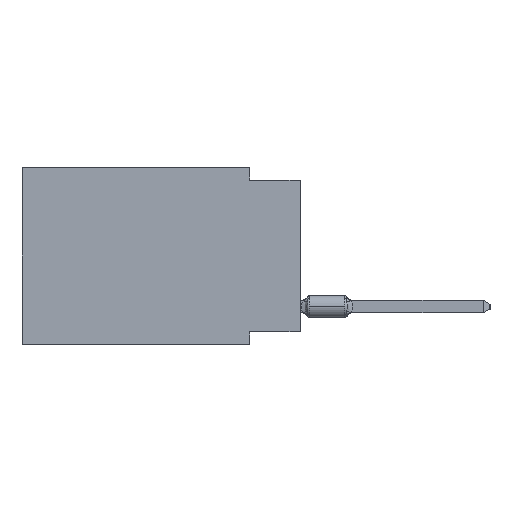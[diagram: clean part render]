
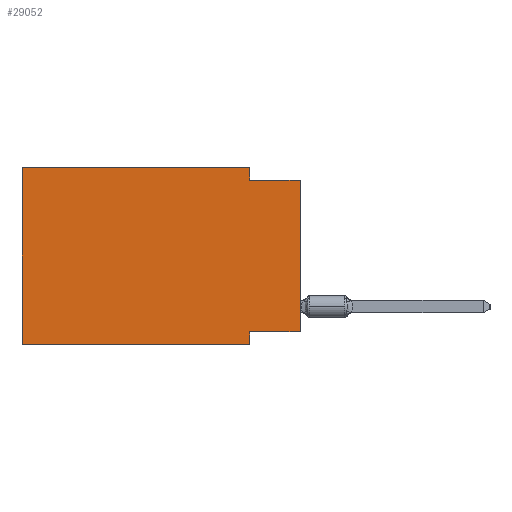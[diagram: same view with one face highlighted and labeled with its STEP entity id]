
A CAD part, left-side view. The second image highlights one B-rep face of the part: STEP entity #29052.
In plain terms, the highlighted planar face has unit normal (-1, 0, 0).
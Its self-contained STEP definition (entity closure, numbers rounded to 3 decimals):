
#316 = DIRECTION ( 'NONE',  ( 0., -1., 0. ) ) ;
#3468 = EDGE_CURVE ( 'NONE', #83949, #24442, #83530, .T. ) ;
#3730 = VERTEX_POINT ( 'NONE', #81602 ) ;
#4729 = EDGE_LOOP ( 'NONE', ( #78545, #19273, #7507, #60123, #86718, #85081, #77925, #61655 ) ) ;
#7156 = VERTEX_POINT ( 'NONE', #19546 ) ;
#7507 = ORIENTED_EDGE ( 'NONE', *, *, #25773, .F. ) ;
#7607 = EDGE_CURVE ( 'NONE', #8416, #3730, #48174, .T. ) ;
#8416 = VERTEX_POINT ( 'NONE', #82884 ) ;
#12441 = VECTOR ( 'NONE', #73471, 1000. ) ;
#12655 = EDGE_CURVE ( 'NONE', #71106, #7156, #22625, .T. ) ;
#12844 = CARTESIAN_POINT ( 'NONE',  ( 0., 2.54, -0.635 ) ) ;
#13614 = VECTOR ( 'NONE', #21148, 1000. ) ;
#15082 = CARTESIAN_POINT ( 'NONE',  ( 0., 0., -8.255 ) ) ;
#16675 = CARTESIAN_POINT ( 'NONE',  ( 0., 2.54, -8.89 ) ) ;
#18164 = LINE ( 'NONE', #24214, #45524 ) ;
#19273 = ORIENTED_EDGE ( 'NONE', *, *, #74665, .F. ) ;
#19546 = CARTESIAN_POINT ( 'NONE',  ( 0., 2.54, 0. ) ) ;
#21148 = DIRECTION ( 'NONE',  ( 0., 1., 0. ) ) ;
#21368 = VECTOR ( 'NONE', #70034, 1000. ) ;
#22625 = LINE ( 'NONE', #49651, #82276 ) ;
#22646 = FACE_OUTER_BOUND ( 'NONE', #4729, .T. ) ;
#23125 = PLANE ( 'NONE',  #54576 ) ;
#23143 = VECTOR ( 'NONE', #34197, 1000. ) ;
#23569 = CARTESIAN_POINT ( 'NONE',  ( 0., 13.97, 0. ) ) ;
#24214 = CARTESIAN_POINT ( 'NONE',  ( 0., 0., -0.635 ) ) ;
#24442 = VERTEX_POINT ( 'NONE', #63668 ) ;
#25773 = EDGE_CURVE ( 'NONE', #7156, #33038, #77188, .T. ) ;
#27216 = CARTESIAN_POINT ( 'NONE',  ( 0., 13.97, -8.89 ) ) ;
#29052 = ADVANCED_FACE ( 'NONE', ( #22646 ), #23125, .F. ) ;
#30479 = DIRECTION ( 'NONE',  ( 0., 0., 1. ) ) ;
#33038 = VERTEX_POINT ( 'NONE', #12844 ) ;
#34197 = DIRECTION ( 'NONE',  ( 0., -1., 0. ) ) ;
#37102 = DIRECTION ( 'NONE',  ( 0., 0., -1. ) ) ;
#41013 = CARTESIAN_POINT ( 'NONE',  ( 0., 0., -8.255 ) ) ;
#44602 = LINE ( 'NONE', #16675, #12441 ) ;
#45524 = VECTOR ( 'NONE', #53079, 1000. ) ;
#48174 = LINE ( 'NONE', #27216, #23143 ) ;
#49651 = CARTESIAN_POINT ( 'NONE',  ( 0., 13.97, 0. ) ) ;
#50788 = VERTEX_POINT ( 'NONE', #51064 ) ;
#51049 = DIRECTION ( 'NONE',  ( 1., 0., 0. ) ) ;
#51064 = CARTESIAN_POINT ( 'NONE',  ( 0., 2.54, -8.255 ) ) ;
#53079 = DIRECTION ( 'NONE',  ( 0., -1., 0. ) ) ;
#54576 = AXIS2_PLACEMENT_3D ( 'NONE', #23569, #51049, #79450 ) ;
#55616 = CARTESIAN_POINT ( 'NONE',  ( 0., 0., 0. ) ) ;
#58621 = VECTOR ( 'NONE', #37102, 1000. ) ;
#58983 = EDGE_CURVE ( 'NONE', #50788, #3730, #44602, .T. ) ;
#60123 = ORIENTED_EDGE ( 'NONE', *, *, #12655, .F. ) ;
#61453 = CARTESIAN_POINT ( 'NONE',  ( 0., 13.97, 0. ) ) ;
#61655 = ORIENTED_EDGE ( 'NONE', *, *, #79797, .F. ) ;
#63668 = CARTESIAN_POINT ( 'NONE',  ( 0., 0., -0.635 ) ) ;
#64074 = EDGE_CURVE ( 'NONE', #8416, #71106, #82098, .T. ) ;
#70034 = DIRECTION ( 'NONE',  ( 0., 0., 1. ) ) ;
#71106 = VERTEX_POINT ( 'NONE', #61453 ) ;
#73471 = DIRECTION ( 'NONE',  ( 0., 0., -1. ) ) ;
#74665 = EDGE_CURVE ( 'NONE', #33038, #24442, #18164, .T. ) ;
#74686 = VECTOR ( 'NONE', #30479, 1000. ) ;
#77188 = LINE ( 'NONE', #79947, #58621 ) ;
#77925 = ORIENTED_EDGE ( 'NONE', *, *, #58983, .F. ) ;
#77949 = LINE ( 'NONE', #15082, #13614 ) ;
#78545 = ORIENTED_EDGE ( 'NONE', *, *, #3468, .T. ) ;
#79450 = DIRECTION ( 'NONE',  ( 0., 0., -1. ) ) ;
#79797 = EDGE_CURVE ( 'NONE', #83949, #50788, #77949, .T. ) ;
#79947 = CARTESIAN_POINT ( 'NONE',  ( 0., 2.54, 0. ) ) ;
#81602 = CARTESIAN_POINT ( 'NONE',  ( 0., 2.54, -8.89 ) ) ;
#81644 = CARTESIAN_POINT ( 'NONE',  ( 0., 13.97, 0. ) ) ;
#82098 = LINE ( 'NONE', #81644, #74686 ) ;
#82276 = VECTOR ( 'NONE', #316, 1000. ) ;
#82884 = CARTESIAN_POINT ( 'NONE',  ( 0., 13.97, -8.89 ) ) ;
#83530 = LINE ( 'NONE', #55616, #21368 ) ;
#83949 = VERTEX_POINT ( 'NONE', #41013 ) ;
#85081 = ORIENTED_EDGE ( 'NONE', *, *, #7607, .T. ) ;
#86718 = ORIENTED_EDGE ( 'NONE', *, *, #64074, .F. ) ;
